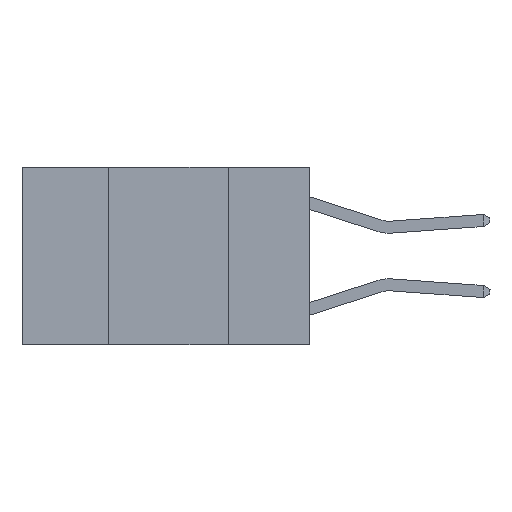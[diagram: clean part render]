
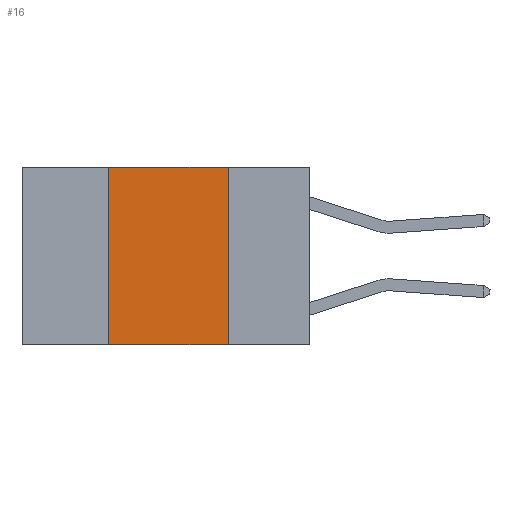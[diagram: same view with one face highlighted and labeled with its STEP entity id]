
A CAD part, left-side view. The second image highlights one B-rep face of the part: STEP entity #16.
In plain terms, the highlighted planar face has unit normal (-1, 0, 0).
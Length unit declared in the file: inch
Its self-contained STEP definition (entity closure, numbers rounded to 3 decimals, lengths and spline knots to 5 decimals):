
#16 = ADVANCED_FACE ( 'NONE', ( #9285 ), #1257, .F. ) ;
#232 = ORIENTED_EDGE ( 'NONE', *, *, #3377, .T. ) ;
#1080 = ORIENTED_EDGE ( 'NONE', *, *, #5458, .F. ) ;
#1160 = VECTOR ( 'NONE', #4966, 39.37008 ) ;
#1257 = PLANE ( 'NONE',  #6265 ) ;
#1346 = VERTEX_POINT ( 'NONE', #4615 ) ;
#1388 = EDGE_CURVE ( 'NONE', #1346, #9862, #11632, .T. ) ;
#1567 = VECTOR ( 'NONE', #2041, 39.37008 ) ;
#1787 = ORIENTED_EDGE ( 'NONE', *, *, #6771, .F. ) ;
#2037 = EDGE_LOOP ( 'NONE', ( #4104, #1080, #1787, #232 ) ) ;
#2041 = DIRECTION ( 'NONE',  ( 0., -1., 0. ) ) ;
#2415 = DIRECTION ( 'NONE',  ( 0., 0., -1. ) ) ;
#2819 = CARTESIAN_POINT ( 'NONE',  ( 0., 0.6, -0.37 ) ) ;
#2907 = VERTEX_POINT ( 'NONE', #10967 ) ;
#3160 = CARTESIAN_POINT ( 'NONE',  ( 0., 0.6, 0. ) ) ;
#3377 = EDGE_CURVE ( 'NONE', #5877, #9862, #12361, .T. ) ;
#3610 = CARTESIAN_POINT ( 'NONE',  ( 0., 0.42, -0.37 ) ) ;
#3955 = CARTESIAN_POINT ( 'NONE',  ( 0., 0.42, 0. ) ) ;
#4104 = ORIENTED_EDGE ( 'NONE', *, *, #1388, .F. ) ;
#4197 = LINE ( 'NONE', #3955, #1160 ) ;
#4615 = CARTESIAN_POINT ( 'NONE',  ( 0., 0.17, 0. ) ) ;
#4966 = DIRECTION ( 'NONE',  ( 0., 0., 1. ) ) ;
#5458 = EDGE_CURVE ( 'NONE', #2907, #1346, #11365, .T. ) ;
#5473 = DIRECTION ( 'NONE',  ( 1., 0., 0. ) ) ;
#5877 = VERTEX_POINT ( 'NONE', #3610 ) ;
#6265 = AXIS2_PLACEMENT_3D ( 'NONE', #3160, #5473, #12632 ) ;
#6771 = EDGE_CURVE ( 'NONE', #5877, #2907, #4197, .T. ) ;
#8595 = VECTOR ( 'NONE', #2415, 39.37008 ) ;
#9285 = FACE_OUTER_BOUND ( 'NONE', #2037, .T. ) ;
#9862 = VERTEX_POINT ( 'NONE', #11241 ) ;
#10773 = CARTESIAN_POINT ( 'NONE',  ( 0., 0.6, 0. ) ) ;
#10967 = CARTESIAN_POINT ( 'NONE',  ( 0., 0.42, 0. ) ) ;
#11241 = CARTESIAN_POINT ( 'NONE',  ( 0., 0.17, -0.37 ) ) ;
#11365 = LINE ( 'NONE', #10773, #11696 ) ;
#11632 = LINE ( 'NONE', #12000, #8595 ) ;
#11696 = VECTOR ( 'NONE', #11810, 39.37008 ) ;
#11810 = DIRECTION ( 'NONE',  ( 0., -1., 0. ) ) ;
#12000 = CARTESIAN_POINT ( 'NONE',  ( 0., 0.17, 0. ) ) ;
#12361 = LINE ( 'NONE', #2819, #1567 ) ;
#12632 = DIRECTION ( 'NONE',  ( 0., 0., -1. ) ) ;
